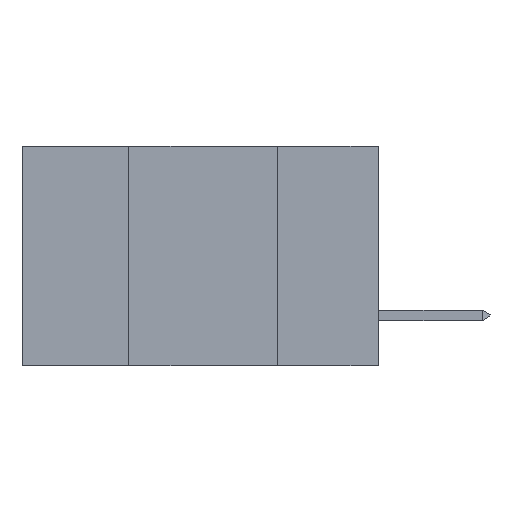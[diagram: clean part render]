
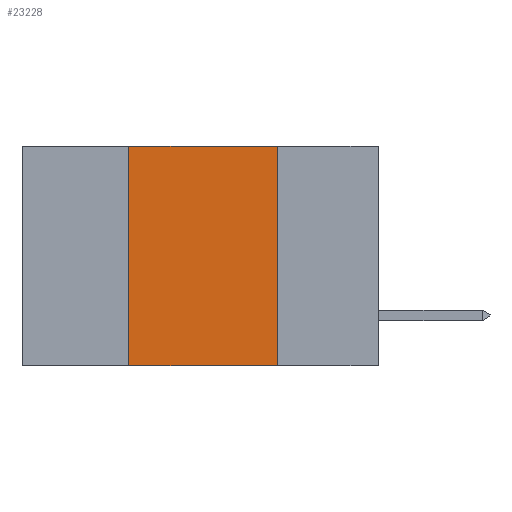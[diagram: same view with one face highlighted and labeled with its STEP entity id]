
A CAD part, left-side view. The second image highlights one B-rep face of the part: STEP entity #23228.
In plain terms, the highlighted planar face has unit normal (-1, 0, 0).
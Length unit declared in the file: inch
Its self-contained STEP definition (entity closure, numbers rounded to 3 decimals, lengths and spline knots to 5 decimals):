
#189 = CARTESIAN_POINT ( 'NONE',  ( 0., 0.42, 0. ) ) ;
#625 = VERTEX_POINT ( 'NONE', #189 ) ;
#1075 = VERTEX_POINT ( 'NONE', #10421 ) ;
#1416 = LINE ( 'NONE', #13111, #22845 ) ;
#2058 = DIRECTION ( 'NONE',  ( 0., 0., -1. ) ) ;
#3457 = ORIENTED_EDGE ( 'NONE', *, *, #13540, .F. ) ;
#3598 = VERTEX_POINT ( 'NONE', #4696 ) ;
#4696 = CARTESIAN_POINT ( 'NONE',  ( 0., 0.42, -0.37 ) ) ;
#5822 = VERTEX_POINT ( 'NONE', #13174 ) ;
#7966 = ORIENTED_EDGE ( 'NONE', *, *, #10746, .F. ) ;
#8344 = EDGE_CURVE ( 'NONE', #5822, #1075, #15953, .T. ) ;
#8374 = FACE_OUTER_BOUND ( 'NONE', #12069, .T. ) ;
#8452 = LINE ( 'NONE', #20340, #16750 ) ;
#8699 = ORIENTED_EDGE ( 'NONE', *, *, #8344, .F. ) ;
#10212 = CARTESIAN_POINT ( 'NONE',  ( 0., 0.6, -0.37 ) ) ;
#10421 = CARTESIAN_POINT ( 'NONE',  ( 0., 0.17, -0.37 ) ) ;
#10746 = EDGE_CURVE ( 'NONE', #3598, #625, #1416, .T. ) ;
#12069 = EDGE_LOOP ( 'NONE', ( #8699, #3457, #7966, #25099 ) ) ;
#12362 = PLANE ( 'NONE',  #17404 ) ;
#13111 = CARTESIAN_POINT ( 'NONE',  ( 0., 0.42, -0.37 ) ) ;
#13174 = CARTESIAN_POINT ( 'NONE',  ( 0., 0.17, 0. ) ) ;
#13540 = EDGE_CURVE ( 'NONE', #625, #5822, #8452, .T. ) ;
#14682 = DIRECTION ( 'NONE',  ( 0., 0., -1. ) ) ;
#15059 = DIRECTION ( 'NONE',  ( 1., 0., 0. ) ) ;
#15953 = LINE ( 'NONE', #19828, #22809 ) ;
#16090 = VECTOR ( 'NONE', #18090, 39.37008 ) ;
#16457 = DIRECTION ( 'NONE',  ( 0., -1., 0. ) ) ;
#16750 = VECTOR ( 'NONE', #16457, 39.37008 ) ;
#17404 = AXIS2_PLACEMENT_3D ( 'NONE', #24120, #15059, #14682 ) ;
#17941 = EDGE_CURVE ( 'NONE', #3598, #1075, #22097, .T. ) ;
#18090 = DIRECTION ( 'NONE',  ( 0., -1., 0. ) ) ;
#19828 = CARTESIAN_POINT ( 'NONE',  ( 0., 0.17, -0.37 ) ) ;
#20340 = CARTESIAN_POINT ( 'NONE',  ( 0., 0.6, 0. ) ) ;
#22097 = LINE ( 'NONE', #10212, #16090 ) ;
#22809 = VECTOR ( 'NONE', #2058, 39.37008 ) ;
#22845 = VECTOR ( 'NONE', #22941, 39.37008 ) ;
#22941 = DIRECTION ( 'NONE',  ( 0., 0., 1. ) ) ;
#23228 = ADVANCED_FACE ( 'NONE', ( #8374 ), #12362, .F. ) ;
#24120 = CARTESIAN_POINT ( 'NONE',  ( 0., 0.6, 0. ) ) ;
#25099 = ORIENTED_EDGE ( 'NONE', *, *, #17941, .T. ) ;
